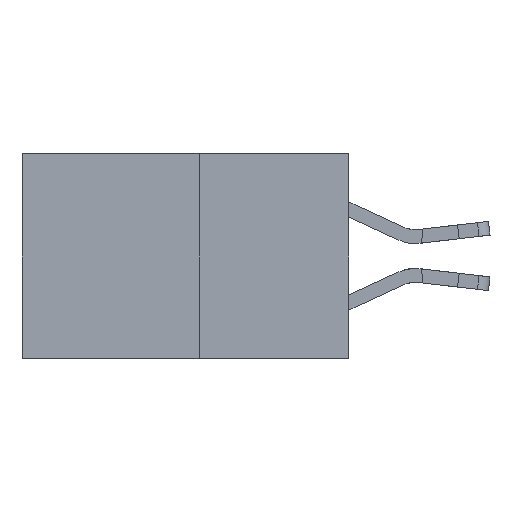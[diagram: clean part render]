
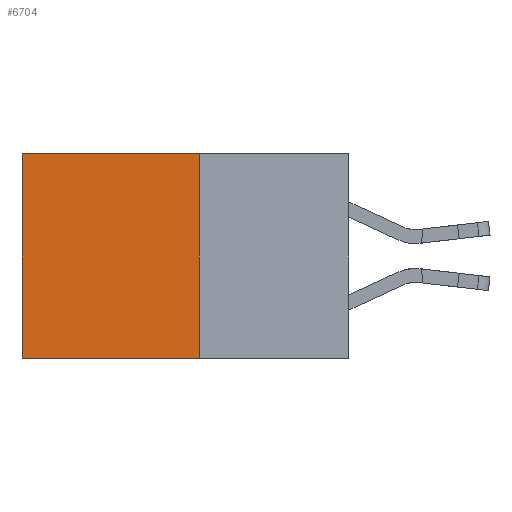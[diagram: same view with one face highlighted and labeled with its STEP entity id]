
A CAD part, left-side view. The second image highlights one B-rep face of the part: STEP entity #6704.
In plain terms, the highlighted planar face has unit normal (-1, 0, 0).
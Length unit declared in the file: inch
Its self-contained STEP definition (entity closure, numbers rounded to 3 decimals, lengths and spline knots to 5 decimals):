
#411 = VERTEX_POINT ( 'NONE', #21117 ) ;
#965 = DIRECTION ( 'NONE',  ( 0., 0., -1. ) ) ;
#1047 = DIRECTION ( 'NONE',  ( 1., 0., 0. ) ) ;
#2202 = AXIS2_PLACEMENT_3D ( 'NONE', #3500, #1047, #965 ) ;
#3141 = ORIENTED_EDGE ( 'NONE', *, *, #9701, .F. ) ;
#3478 = PLANE ( 'NONE',  #2202 ) ;
#3500 = CARTESIAN_POINT ( 'NONE',  ( 0.277, 0.27, -0.37 ) ) ;
#3944 = FACE_OUTER_BOUND ( 'NONE', #6993, .T. ) ;
#5474 = VECTOR ( 'NONE', #25714, 39.37008 ) ;
#6704 = ADVANCED_FACE ( 'NONE', ( #3944 ), #3478, .F. ) ;
#6993 = EDGE_LOOP ( 'NONE', ( #21257, #3141, #16906, #23068 ) ) ;
#7501 = EDGE_CURVE ( 'NONE', #25568, #10846, #10238, .T. ) ;
#7834 = DIRECTION ( 'NONE',  ( 0., 0., -1. ) ) ;
#9284 = DIRECTION ( 'NONE',  ( 0., 0., -1. ) ) ;
#9701 = EDGE_CURVE ( 'NONE', #17054, #10846, #10754, .T. ) ;
#10238 = LINE ( 'NONE', #17103, #25539 ) ;
#10263 = LINE ( 'NONE', #11474, #20319 ) ;
#10754 = LINE ( 'NONE', #17747, #5474 ) ;
#10846 = VERTEX_POINT ( 'NONE', #21643 ) ;
#11474 = CARTESIAN_POINT ( 'NONE',  ( 0.277, 0.27, 0. ) ) ;
#11864 = CARTESIAN_POINT ( 'NONE',  ( 0.277, 0.27, -0.37 ) ) ;
#14582 = EDGE_CURVE ( 'NONE', #411, #25568, #10263, .T. ) ;
#15013 = CARTESIAN_POINT ( 'NONE',  ( 0.277, 0.27, -0.37 ) ) ;
#15400 = EDGE_CURVE ( 'NONE', #411, #17054, #23376, .T. ) ;
#16906 = ORIENTED_EDGE ( 'NONE', *, *, #15400, .F. ) ;
#17054 = VERTEX_POINT ( 'NONE', #15013 ) ;
#17103 = CARTESIAN_POINT ( 'NONE',  ( 0.277, 0.59, -0.37 ) ) ;
#17465 = VECTOR ( 'NONE', #7834, 39.37008 ) ;
#17747 = CARTESIAN_POINT ( 'NONE',  ( 0.277, 0.27, -0.37 ) ) ;
#19890 = CARTESIAN_POINT ( 'NONE',  ( 0.277, 0.59, 0. ) ) ;
#20319 = VECTOR ( 'NONE', #25414, 39.37008 ) ;
#21117 = CARTESIAN_POINT ( 'NONE',  ( 0.277, 0.27, 0. ) ) ;
#21257 = ORIENTED_EDGE ( 'NONE', *, *, #7501, .T. ) ;
#21643 = CARTESIAN_POINT ( 'NONE',  ( 0.277, 0.59, -0.37 ) ) ;
#23068 = ORIENTED_EDGE ( 'NONE', *, *, #14582, .T. ) ;
#23376 = LINE ( 'NONE', #11864, #17465 ) ;
#25414 = DIRECTION ( 'NONE',  ( 0., 1., 0. ) ) ;
#25539 = VECTOR ( 'NONE', #9284, 39.37008 ) ;
#25568 = VERTEX_POINT ( 'NONE', #19890 ) ;
#25714 = DIRECTION ( 'NONE',  ( 0., 1., 0. ) ) ;
